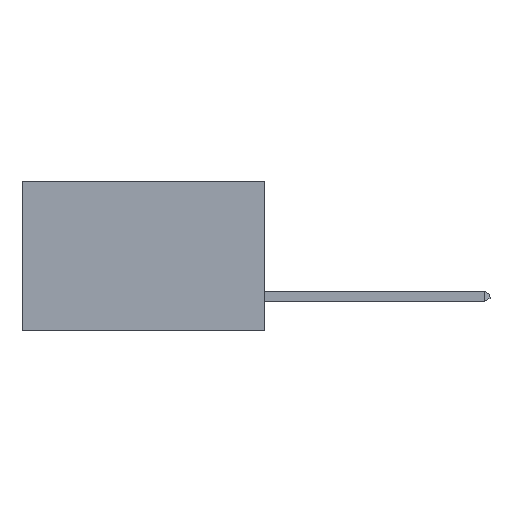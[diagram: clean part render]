
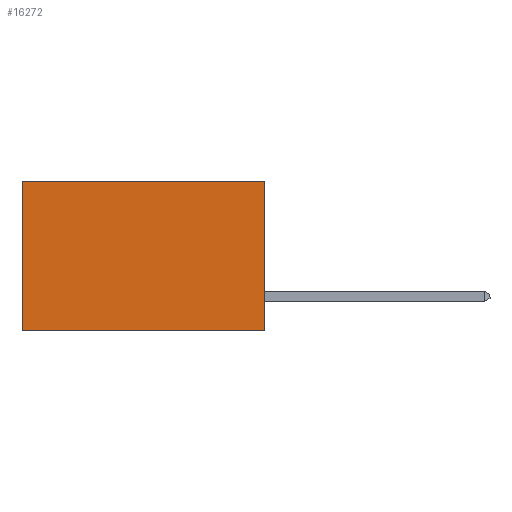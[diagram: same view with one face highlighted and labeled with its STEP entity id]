
A CAD part, left-side view. The second image highlights one B-rep face of the part: STEP entity #16272.
In plain terms, the highlighted planar face has unit normal (-1, 0, 0).
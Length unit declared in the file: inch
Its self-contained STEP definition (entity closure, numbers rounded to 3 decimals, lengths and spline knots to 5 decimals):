
#262 = DIRECTION ( 'NONE',  ( 0., 0., -1. ) ) ;
#869 = ORIENTED_EDGE ( 'NONE', *, *, #11343, .T. ) ;
#1759 = VERTEX_POINT ( 'NONE', #10529 ) ;
#2211 = DIRECTION ( 'NONE',  ( 0., 1., 0. ) ) ;
#2238 = CARTESIAN_POINT ( 'NONE',  ( 0.298, 0., -0.37 ) ) ;
#2396 = VERTEX_POINT ( 'NONE', #15062 ) ;
#2638 = CARTESIAN_POINT ( 'NONE',  ( 0.298, 0., 0. ) ) ;
#2728 = DIRECTION ( 'NONE',  ( 0., 1., 0. ) ) ;
#3096 = EDGE_LOOP ( 'NONE', ( #8284, #7763, #8768, #869 ) ) ;
#4187 = LINE ( 'NONE', #17414, #7306 ) ;
#7239 = EDGE_CURVE ( 'NONE', #9450, #2396, #4187, .T. ) ;
#7306 = VECTOR ( 'NONE', #14925, 39.37008 ) ;
#7664 = EDGE_CURVE ( 'NONE', #1759, #9002, #15182, .T. ) ;
#7763 = ORIENTED_EDGE ( 'NONE', *, *, #13234, .F. ) ;
#7987 = CARTESIAN_POINT ( 'NONE',  ( 0.298, 0., 0. ) ) ;
#8284 = ORIENTED_EDGE ( 'NONE', *, *, #7664, .T. ) ;
#8698 = LINE ( 'NONE', #2638, #15175 ) ;
#8768 = ORIENTED_EDGE ( 'NONE', *, *, #7239, .F. ) ;
#9002 = VERTEX_POINT ( 'NONE', #18640 ) ;
#9450 = VERTEX_POINT ( 'NONE', #10578 ) ;
#9505 = DIRECTION ( 'NONE',  ( 1., 0., 0. ) ) ;
#9819 = CARTESIAN_POINT ( 'NONE',  ( 0.298, 0.6, 0. ) ) ;
#10067 = AXIS2_PLACEMENT_3D ( 'NONE', #7987, #9505, #262 ) ;
#10529 = CARTESIAN_POINT ( 'NONE',  ( 0.298, 0.6, 0. ) ) ;
#10578 = CARTESIAN_POINT ( 'NONE',  ( 0.298, 0., 0. ) ) ;
#11276 = VECTOR ( 'NONE', #16750, 39.37008 ) ;
#11343 = EDGE_CURVE ( 'NONE', #9450, #1759, #8698, .T. ) ;
#13234 = EDGE_CURVE ( 'NONE', #2396, #9002, #19031, .T. ) ;
#14925 = DIRECTION ( 'NONE',  ( 0., 0., -1. ) ) ;
#15062 = CARTESIAN_POINT ( 'NONE',  ( 0.298, 0., -0.37 ) ) ;
#15175 = VECTOR ( 'NONE', #2728, 39.37008 ) ;
#15182 = LINE ( 'NONE', #9819, #11276 ) ;
#16272 = ADVANCED_FACE ( 'NONE', ( #16482 ), #16793, .F. ) ;
#16482 = FACE_OUTER_BOUND ( 'NONE', #3096, .T. ) ;
#16750 = DIRECTION ( 'NONE',  ( 0., 0., -1. ) ) ;
#16793 = PLANE ( 'NONE',  #10067 ) ;
#17414 = CARTESIAN_POINT ( 'NONE',  ( 0.298, 0., 0. ) ) ;
#18618 = VECTOR ( 'NONE', #2211, 39.37008 ) ;
#18640 = CARTESIAN_POINT ( 'NONE',  ( 0.298, 0.6, -0.37 ) ) ;
#19031 = LINE ( 'NONE', #2238, #18618 ) ;
